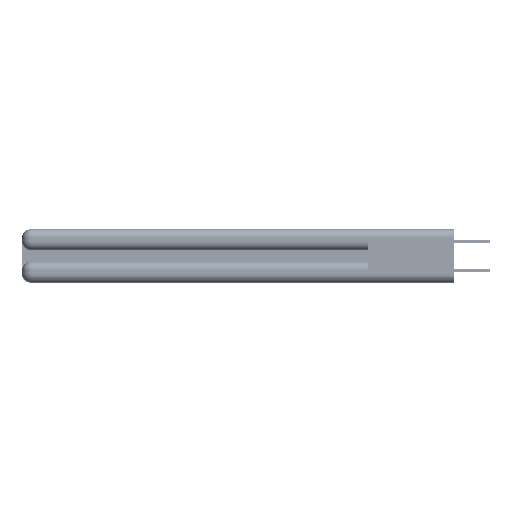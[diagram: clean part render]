
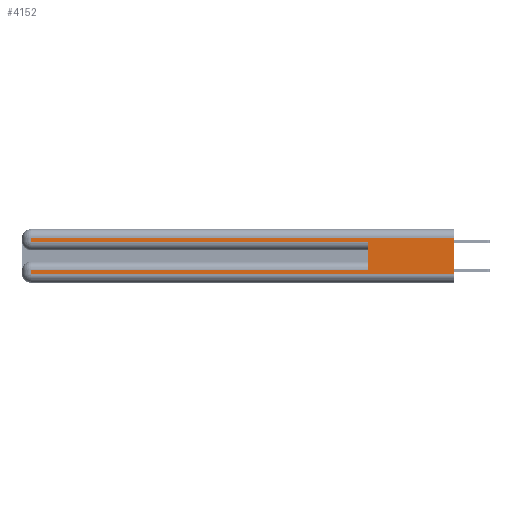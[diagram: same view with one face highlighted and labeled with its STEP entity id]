
A CAD part, left-side view. The second image highlights one B-rep face of the part: STEP entity #4152.
In plain terms, the highlighted planar face has unit normal (-1, 0, 0).
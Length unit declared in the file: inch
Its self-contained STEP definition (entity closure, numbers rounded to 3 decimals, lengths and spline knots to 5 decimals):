
#1707 = ORIENTED_EDGE ( 'NONE', *, *, #21509, .T. ) ;
#2541 = DIRECTION ( 'NONE',  ( 0., 0., 1. ) ) ;
#3332 = LINE ( 'NONE', #41911, #32680 ) ;
#3594 = CARTESIAN_POINT ( 'NONE',  ( 0., 0., 0.085 ) ) ;
#4152 = ADVANCED_FACE ( 'NONE', ( #32477 ), #29921, .F. ) ;
#5394 = EDGE_LOOP ( 'NONE', ( #33608, #35361, #1707, #8780, #31725, #30025, #36242, #6240 ) ) ;
#6060 = LINE ( 'NONE', #44073, #33216 ) ;
#6240 = ORIENTED_EDGE ( 'NONE', *, *, #26333, .T. ) ;
#6441 = CARTESIAN_POINT ( 'NONE',  ( 0., 0., 0.31 ) ) ;
#6794 = VECTOR ( 'NONE', #27376, 39.37008 ) ;
#6864 = LINE ( 'NONE', #27012, #34094 ) ;
#7548 = EDGE_CURVE ( 'NONE', #22979, #30910, #6060, .T. ) ;
#8544 = DIRECTION ( 'NONE',  ( 0., 0., -1. ) ) ;
#8780 = ORIENTED_EDGE ( 'NONE', *, *, #7548, .T. ) ;
#9261 = CARTESIAN_POINT ( 'NONE',  ( 0., 0., 0.31 ) ) ;
#9704 = DIRECTION ( 'NONE',  ( 0., 0., -1. ) ) ;
#10270 = DIRECTION ( 'NONE',  ( 0., 0., -1. ) ) ;
#10732 = CARTESIAN_POINT ( 'NONE',  ( 0., 0.6, 0.085 ) ) ;
#11735 = EDGE_CURVE ( 'NONE', #11907, #14185, #36121, .T. ) ;
#11907 = VERTEX_POINT ( 'NONE', #22343 ) ;
#12327 = LINE ( 'NONE', #29209, #37921 ) ;
#12889 = LINE ( 'NONE', #9261, #6794 ) ;
#13039 = VERTEX_POINT ( 'NONE', #24351 ) ;
#14038 = VECTOR ( 'NONE', #23846, 39.37008 ) ;
#14185 = VERTEX_POINT ( 'NONE', #19928 ) ;
#14189 = VECTOR ( 'NONE', #40334, 39.37008 ) ;
#14546 = LINE ( 'NONE', #41237, #14038 ) ;
#15551 = EDGE_CURVE ( 'NONE', #38272, #11907, #29715, .T. ) ;
#16748 = VERTEX_POINT ( 'NONE', #36994 ) ;
#17132 = CARTESIAN_POINT ( 'NONE',  ( 0., 2.94, 0.37 ) ) ;
#18733 = CARTESIAN_POINT ( 'NONE',  ( 0., 0., 0.37 ) ) ;
#19928 = CARTESIAN_POINT ( 'NONE',  ( 0., 2.94, 0.06 ) ) ;
#21509 = EDGE_CURVE ( 'NONE', #16748, #22979, #12327, .T. ) ;
#22343 = CARTESIAN_POINT ( 'NONE',  ( 0., 2.94, 0.085 ) ) ;
#22476 = EDGE_CURVE ( 'NONE', #31063, #16748, #12889, .T. ) ;
#22864 = CARTESIAN_POINT ( 'NONE',  ( 0., 2.94, 0.285 ) ) ;
#22979 = VERTEX_POINT ( 'NONE', #22864 ) ;
#23035 = CARTESIAN_POINT ( 'NONE',  ( 0., 0.6, 0.285 ) ) ;
#23846 = DIRECTION ( 'NONE',  ( 0., -1., 0. ) ) ;
#24351 = CARTESIAN_POINT ( 'NONE',  ( 0., 0., 0.06 ) ) ;
#26333 = EDGE_CURVE ( 'NONE', #14185, #13039, #14546, .T. ) ;
#27012 = CARTESIAN_POINT ( 'NONE',  ( 0., 0.6, 0.145 ) ) ;
#27376 = DIRECTION ( 'NONE',  ( 0., 1., 0. ) ) ;
#29209 = CARTESIAN_POINT ( 'NONE',  ( 0., 2.94, 0.37 ) ) ;
#29715 = LINE ( 'NONE', #3594, #14189 ) ;
#29921 = PLANE ( 'NONE',  #41385 ) ;
#30025 = ORIENTED_EDGE ( 'NONE', *, *, #15551, .T. ) ;
#30910 = VERTEX_POINT ( 'NONE', #23035 ) ;
#31063 = VERTEX_POINT ( 'NONE', #6441 ) ;
#31725 = ORIENTED_EDGE ( 'NONE', *, *, #34701, .F. ) ;
#32477 = FACE_OUTER_BOUND ( 'NONE', #5394, .T. ) ;
#32680 = VECTOR ( 'NONE', #10270, 39.37008 ) ;
#33216 = VECTOR ( 'NONE', #38713, 39.37008 ) ;
#33509 = DIRECTION ( 'NONE',  ( 1., 0., 0. ) ) ;
#33608 = ORIENTED_EDGE ( 'NONE', *, *, #45681, .F. ) ;
#34094 = VECTOR ( 'NONE', #2541, 39.37008 ) ;
#34701 = EDGE_CURVE ( 'NONE', #38272, #30910, #6864, .T. ) ;
#35361 = ORIENTED_EDGE ( 'NONE', *, *, #22476, .T. ) ;
#36076 = DIRECTION ( 'NONE',  ( 0., 0., -1. ) ) ;
#36121 = LINE ( 'NONE', #17132, #37865 ) ;
#36242 = ORIENTED_EDGE ( 'NONE', *, *, #11735, .T. ) ;
#36994 = CARTESIAN_POINT ( 'NONE',  ( 0., 2.94, 0.31 ) ) ;
#37865 = VECTOR ( 'NONE', #9704, 39.37008 ) ;
#37921 = VECTOR ( 'NONE', #36076, 39.37008 ) ;
#38272 = VERTEX_POINT ( 'NONE', #10732 ) ;
#38713 = DIRECTION ( 'NONE',  ( 0., -1., 0. ) ) ;
#40334 = DIRECTION ( 'NONE',  ( 0., 1., 0. ) ) ;
#41237 = CARTESIAN_POINT ( 'NONE',  ( 0., 0., 0.06 ) ) ;
#41385 = AXIS2_PLACEMENT_3D ( 'NONE', #18733, #33509, #8544 ) ;
#41911 = CARTESIAN_POINT ( 'NONE',  ( 0., 0., 0.37 ) ) ;
#44073 = CARTESIAN_POINT ( 'NONE',  ( 0., 0., 0.285 ) ) ;
#45681 = EDGE_CURVE ( 'NONE', #31063, #13039, #3332, .T. ) ;
